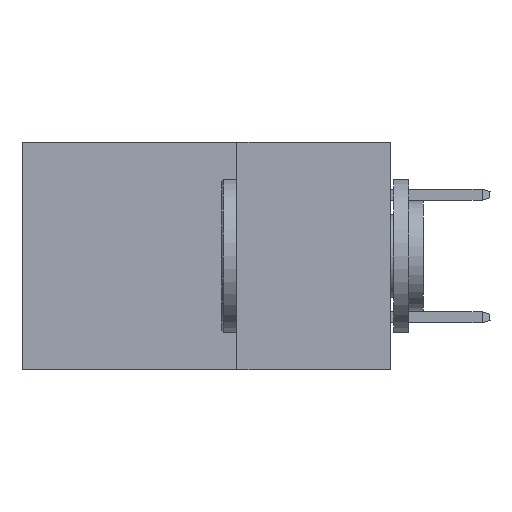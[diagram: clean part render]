
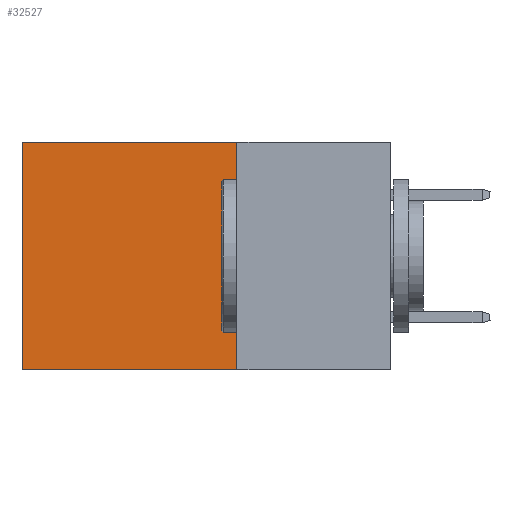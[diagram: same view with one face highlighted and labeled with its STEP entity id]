
A CAD part, left-side view. The second image highlights one B-rep face of the part: STEP entity #32527.
In plain terms, the highlighted planar face has unit normal (-1, 0, 0).
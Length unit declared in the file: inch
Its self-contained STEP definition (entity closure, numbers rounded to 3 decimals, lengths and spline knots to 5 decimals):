
#245 = DIRECTION ( 'NONE',  ( 0., 0., -1. ) ) ;
#796 = CARTESIAN_POINT ( 'NONE',  ( 0.2875, 0.25, 0. ) ) ;
#839 = VERTEX_POINT ( 'NONE', #28340 ) ;
#1832 = VERTEX_POINT ( 'NONE', #3691 ) ;
#3414 = VERTEX_POINT ( 'NONE', #18825 ) ;
#3680 = DIRECTION ( 'NONE',  ( 0., 0., -1. ) ) ;
#3691 = CARTESIAN_POINT ( 'NONE',  ( 0.2875, 0.25, -0.37 ) ) ;
#3894 = LINE ( 'NONE', #23099, #7497 ) ;
#4346 = EDGE_CURVE ( 'NONE', #1832, #21595, #21242, .T. ) ;
#6411 = VECTOR ( 'NONE', #35524, 39.37008 ) ;
#7497 = VECTOR ( 'NONE', #20986, 39.37008 ) ;
#9039 = AXIS2_PLACEMENT_3D ( 'NONE', #796, #20867, #3680 ) ;
#12444 = VECTOR ( 'NONE', #26843, 39.37008 ) ;
#13146 = ORIENTED_EDGE ( 'NONE', *, *, #27549, .T. ) ;
#13160 = CARTESIAN_POINT ( 'NONE',  ( 0.2875, 0.6, -0.37 ) ) ;
#15205 = EDGE_CURVE ( 'NONE', #839, #1832, #16477, .T. ) ;
#15500 = CARTESIAN_POINT ( 'NONE',  ( 0.2875, 0.25, -0.37 ) ) ;
#16477 = LINE ( 'NONE', #24205, #12444 ) ;
#17437 = CARTESIAN_POINT ( 'NONE',  ( 0.2875, 0.6, 0. ) ) ;
#18029 = VECTOR ( 'NONE', #245, 39.37008 ) ;
#18825 = CARTESIAN_POINT ( 'NONE',  ( 0.2875, 0.6, 0. ) ) ;
#19623 = EDGE_LOOP ( 'NONE', ( #13146, #30354, #36200, #35729 ) ) ;
#20867 = DIRECTION ( 'NONE',  ( 1., 0., 0. ) ) ;
#20986 = DIRECTION ( 'NONE',  ( 0., 1., 0. ) ) ;
#21242 = LINE ( 'NONE', #15500, #6411 ) ;
#21595 = VERTEX_POINT ( 'NONE', #13160 ) ;
#21966 = FACE_OUTER_BOUND ( 'NONE', #19623, .T. ) ;
#23099 = CARTESIAN_POINT ( 'NONE',  ( 0.2875, 0.25, 0. ) ) ;
#24205 = CARTESIAN_POINT ( 'NONE',  ( 0.2875, 0.25, 0. ) ) ;
#25627 = LINE ( 'NONE', #17437, #18029 ) ;
#26607 = PLANE ( 'NONE',  #9039 ) ;
#26843 = DIRECTION ( 'NONE',  ( 0., 0., -1. ) ) ;
#27549 = EDGE_CURVE ( 'NONE', #3414, #21595, #25627, .T. ) ;
#28340 = CARTESIAN_POINT ( 'NONE',  ( 0.2875, 0.25, 0. ) ) ;
#30354 = ORIENTED_EDGE ( 'NONE', *, *, #4346, .F. ) ;
#32527 = ADVANCED_FACE ( 'NONE', ( #21966 ), #26607, .F. ) ;
#34278 = EDGE_CURVE ( 'NONE', #839, #3414, #3894, .T. ) ;
#35524 = DIRECTION ( 'NONE',  ( 0., 1., 0. ) ) ;
#35729 = ORIENTED_EDGE ( 'NONE', *, *, #34278, .T. ) ;
#36200 = ORIENTED_EDGE ( 'NONE', *, *, #15205, .F. ) ;
